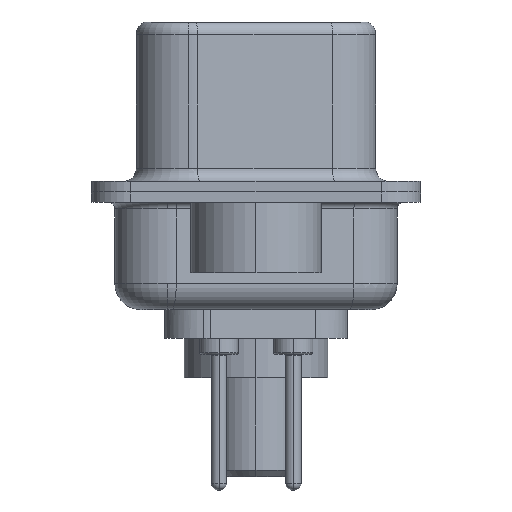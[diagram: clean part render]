
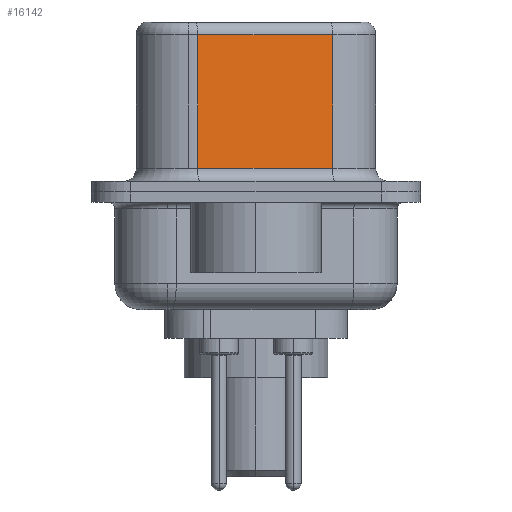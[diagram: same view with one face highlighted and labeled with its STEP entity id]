
A CAD part, left-side view. The second image highlights one B-rep face of the part: STEP entity #16142.
In plain terms, the highlighted planar face has unit normal (-0.985, -0.174, 0).
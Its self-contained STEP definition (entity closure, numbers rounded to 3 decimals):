
#229 = CARTESIAN_POINT ( 'NONE',  ( 3.67, 2.233, 6.02 ) ) ;
#527 = ORIENTED_EDGE ( 'NONE', *, *, #16332, .T. ) ;
#877 = DIRECTION ( 'NONE',  ( 0.985, 0.174, 0. ) ) ;
#995 = CARTESIAN_POINT ( 'NONE',  ( 4.58, -2.927, 6.52 ) ) ;
#1833 = ORIENTED_EDGE ( 'NONE', *, *, #9216, .T. ) ;
#2226 = AXIS2_PLACEMENT_3D ( 'NONE', #12468, #877, #10056 ) ;
#2537 = VERTEX_POINT ( 'NONE', #12476 ) ;
#3303 = EDGE_CURVE ( 'NONE', #8556, #2537, #4526, .T. ) ;
#3466 = VERTEX_POINT ( 'NONE', #229 ) ;
#3582 = DIRECTION ( 'NONE',  ( -0.174, 0.985, 0. ) ) ;
#3600 = LINE ( 'NONE', #14033, #13615 ) ;
#3673 = LINE ( 'NONE', #9830, #10046 ) ;
#3939 = DIRECTION ( 'NONE',  ( 0.174, -0.985, 0. ) ) ;
#4308 = VERTEX_POINT ( 'NONE', #13663 ) ;
#4526 = LINE ( 'NONE', #995, #13331 ) ;
#4863 = CARTESIAN_POINT ( 'NONE',  ( 4.58, -2.927, 6.02 ) ) ;
#6074 = ORIENTED_EDGE ( 'NONE', *, *, #9317, .T. ) ;
#6247 = PLANE ( 'NONE',  #2226 ) ;
#8556 = VERTEX_POINT ( 'NONE', #8930 ) ;
#8930 = CARTESIAN_POINT ( 'NONE',  ( 4.58, -2.927, 6.02 ) ) ;
#9216 = EDGE_CURVE ( 'NONE', #3466, #4308, #3673, .T. ) ;
#9245 = VECTOR ( 'NONE', #3582, 1000. ) ;
#9317 = EDGE_CURVE ( 'NONE', #8556, #3466, #9648, .T. ) ;
#9458 = ORIENTED_EDGE ( 'NONE', *, *, #3303, .F. ) ;
#9648 = LINE ( 'NONE', #4863, #9245 ) ;
#9741 = DIRECTION ( 'NONE',  ( 0., 0., -1. ) ) ;
#9830 = CARTESIAN_POINT ( 'NONE',  ( 3.67, 2.233, 6.52 ) ) ;
#10046 = VECTOR ( 'NONE', #11079, 1000. ) ;
#10056 = DIRECTION ( 'NONE',  ( -0.174, 0.985, 0. ) ) ;
#11079 = DIRECTION ( 'NONE',  ( 0., 0., -1. ) ) ;
#11748 = EDGE_LOOP ( 'NONE', ( #9458, #6074, #1833, #527 ) ) ;
#12468 = CARTESIAN_POINT ( 'NONE',  ( 4.58, -2.927, 6.52 ) ) ;
#12476 = CARTESIAN_POINT ( 'NONE',  ( 4.58, -2.927, 0.9 ) ) ;
#13331 = VECTOR ( 'NONE', #9741, 1000. ) ;
#13615 = VECTOR ( 'NONE', #3939, 1000. ) ;
#13663 = CARTESIAN_POINT ( 'NONE',  ( 3.67, 2.233, 0.9 ) ) ;
#14033 = CARTESIAN_POINT ( 'NONE',  ( 4.58, -2.927, 0.9 ) ) ;
#15245 = FACE_OUTER_BOUND ( 'NONE', #11748, .T. ) ;
#16142 = ADVANCED_FACE ( 'NONE', ( #15245 ), #6247, .F. ) ;
#16332 = EDGE_CURVE ( 'NONE', #4308, #2537, #3600, .T. ) ;
